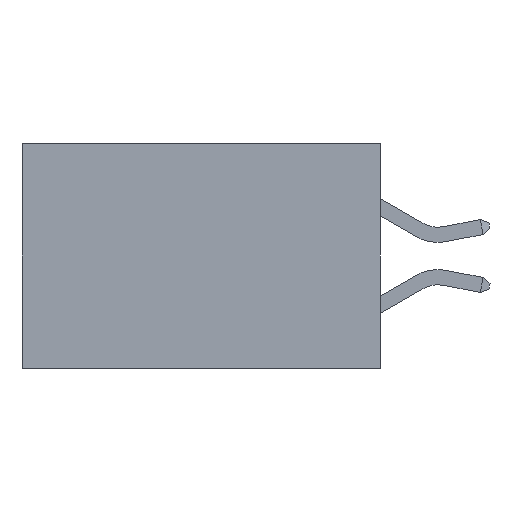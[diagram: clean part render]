
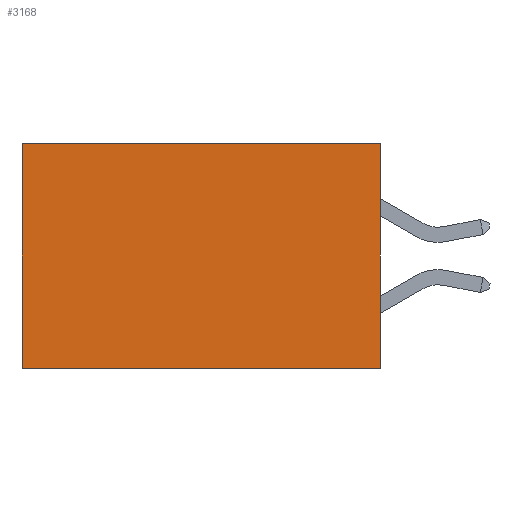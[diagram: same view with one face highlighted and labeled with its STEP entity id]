
A CAD part, left-side view. The second image highlights one B-rep face of the part: STEP entity #3168.
In plain terms, the highlighted planar face has unit normal (-1, 0, 0).
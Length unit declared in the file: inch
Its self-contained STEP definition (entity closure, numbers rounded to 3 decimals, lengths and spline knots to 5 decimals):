
#112 = EDGE_LOOP ( 'NONE', ( #2301, #2320, #2331, #2356 ) ) ;
#618 = DIRECTION ( 'NONE',  ( 0., 0., -1. ) ) ;
#717 = VECTOR ( 'NONE', #5561, 39.37008 ) ;
#868 = CARTESIAN_POINT ( 'NONE',  ( 0.277, 0., -0.37 ) ) ;
#954 = CARTESIAN_POINT ( 'NONE',  ( 0.277, 0.59, -0.37 ) ) ;
#1078 = LINE ( 'NONE', #1185, #3033 ) ;
#1162 = DIRECTION ( 'NONE',  ( 0., 1., 0. ) ) ;
#1185 = CARTESIAN_POINT ( 'NONE',  ( 0.277, 0., 0. ) ) ;
#1187 = VERTEX_POINT ( 'NONE', #4738 ) ;
#1636 = CARTESIAN_POINT ( 'NONE',  ( 0.277, 0.59, -0.37 ) ) ;
#2271 = FACE_OUTER_BOUND ( 'NONE', #112, .T. ) ;
#2301 = ORIENTED_EDGE ( 'NONE', *, *, #5894, .T. ) ;
#2320 = ORIENTED_EDGE ( 'NONE', *, *, #2674, .F. ) ;
#2331 = ORIENTED_EDGE ( 'NONE', *, *, #7240, .F. ) ;
#2356 = ORIENTED_EDGE ( 'NONE', *, *, #4176, .T. ) ;
#2674 = EDGE_CURVE ( 'NONE', #7431, #4242, #7043, .T. ) ;
#3033 = VECTOR ( 'NONE', #1162, 39.37008 ) ;
#3168 = ADVANCED_FACE ( 'NONE', ( #2271 ), #7441, .F. ) ;
#3404 = AXIS2_PLACEMENT_3D ( 'NONE', #868, #7279, #7270 ) ;
#4176 = EDGE_CURVE ( 'NONE', #4632, #1187, #1078, .T. ) ;
#4242 = VERTEX_POINT ( 'NONE', #954 ) ;
#4628 = VECTOR ( 'NONE', #5839, 39.37008 ) ;
#4632 = VERTEX_POINT ( 'NONE', #5055 ) ;
#4738 = CARTESIAN_POINT ( 'NONE',  ( 0.277, 0.59, 0. ) ) ;
#5055 = CARTESIAN_POINT ( 'NONE',  ( 0.277, 0., 0. ) ) ;
#5391 = CARTESIAN_POINT ( 'NONE',  ( 0.277, 0., -0.37 ) ) ;
#5505 = CARTESIAN_POINT ( 'NONE',  ( 0.277, 0., -0.37 ) ) ;
#5561 = DIRECTION ( 'NONE',  ( 0., 1., 0. ) ) ;
#5586 = CARTESIAN_POINT ( 'NONE',  ( 0.277, 0., -0.37 ) ) ;
#5620 = VECTOR ( 'NONE', #618, 39.37008 ) ;
#5832 = LINE ( 'NONE', #1636, #4628 ) ;
#5839 = DIRECTION ( 'NONE',  ( 0., 0., -1. ) ) ;
#5894 = EDGE_CURVE ( 'NONE', #1187, #4242, #5832, .T. ) ;
#7043 = LINE ( 'NONE', #5505, #717 ) ;
#7168 = LINE ( 'NONE', #5391, #5620 ) ;
#7240 = EDGE_CURVE ( 'NONE', #4632, #7431, #7168, .T. ) ;
#7270 = DIRECTION ( 'NONE',  ( 0., 0., -1. ) ) ;
#7279 = DIRECTION ( 'NONE',  ( 1., 0., 0. ) ) ;
#7431 = VERTEX_POINT ( 'NONE', #5586 ) ;
#7441 = PLANE ( 'NONE',  #3404 ) ;
